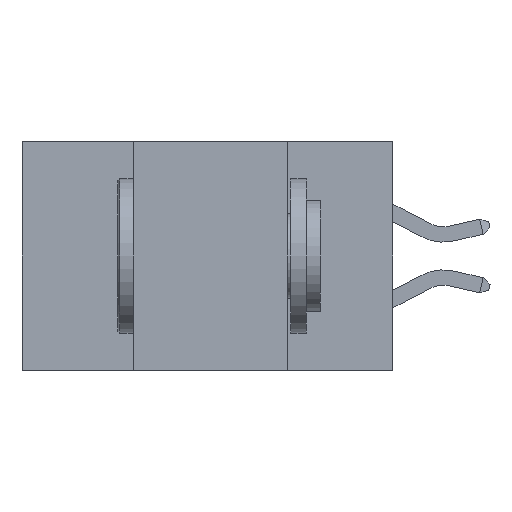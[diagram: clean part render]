
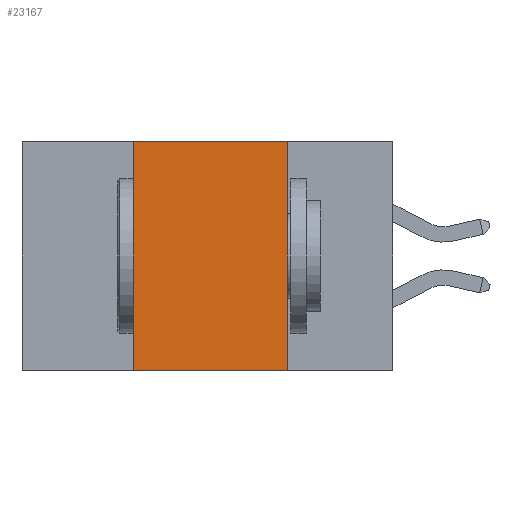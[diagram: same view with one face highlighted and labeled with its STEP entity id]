
A CAD part, left-side view. The second image highlights one B-rep face of the part: STEP entity #23167.
In plain terms, the highlighted planar face has unit normal (-1, 0, 0).
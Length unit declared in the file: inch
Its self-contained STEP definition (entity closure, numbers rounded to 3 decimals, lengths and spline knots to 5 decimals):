
#390 = EDGE_CURVE ( 'NONE', #35558, #11624, #39982, .T. ) ;
#1062 = VERTEX_POINT ( 'NONE', #30200 ) ;
#2316 = DIRECTION ( 'NONE',  ( 0., 0., -1. ) ) ;
#5757 = ORIENTED_EDGE ( 'NONE', *, *, #390, .F. ) ;
#5791 = PLANE ( 'NONE',  #6320 ) ;
#6320 = AXIS2_PLACEMENT_3D ( 'NONE', #9285, #32191, #12576 ) ;
#6738 = DIRECTION ( 'NONE',  ( 0., -1., 0. ) ) ;
#9285 = CARTESIAN_POINT ( 'NONE',  ( 0., 0.6, 0. ) ) ;
#10942 = EDGE_LOOP ( 'NONE', ( #28125, #5757, #19168, #29749 ) ) ;
#11624 = VERTEX_POINT ( 'NONE', #15081 ) ;
#11671 = CARTESIAN_POINT ( 'NONE',  ( 0., 0.17, -0.37 ) ) ;
#12576 = DIRECTION ( 'NONE',  ( 0., 0., -1. ) ) ;
#13021 = DIRECTION ( 'NONE',  ( 0., 0., 1. ) ) ;
#13224 = CARTESIAN_POINT ( 'NONE',  ( 0., 0.6, -0.37 ) ) ;
#13572 = CARTESIAN_POINT ( 'NONE',  ( 0., 0.6, 0. ) ) ;
#15081 = CARTESIAN_POINT ( 'NONE',  ( 0., 0.17, 0. ) ) ;
#15879 = VECTOR ( 'NONE', #13021, 39.37008 ) ;
#17072 = VECTOR ( 'NONE', #6738, 39.37008 ) ;
#17539 = VERTEX_POINT ( 'NONE', #11671 ) ;
#17560 = CARTESIAN_POINT ( 'NONE',  ( 0., 0.42, 0. ) ) ;
#19168 = ORIENTED_EDGE ( 'NONE', *, *, #20174, .F. ) ;
#19744 = CARTESIAN_POINT ( 'NONE',  ( 0., 0.42, 0. ) ) ;
#20174 = EDGE_CURVE ( 'NONE', #1062, #35558, #22017, .T. ) ;
#21080 = VECTOR ( 'NONE', #2316, 39.37008 ) ;
#22017 = LINE ( 'NONE', #19744, #15879 ) ;
#23167 = ADVANCED_FACE ( 'NONE', ( #33604 ), #5791, .F. ) ;
#28125 = ORIENTED_EDGE ( 'NONE', *, *, #39306, .F. ) ;
#29186 = VECTOR ( 'NONE', #33602, 39.37008 ) ;
#29749 = ORIENTED_EDGE ( 'NONE', *, *, #37909, .T. ) ;
#30200 = CARTESIAN_POINT ( 'NONE',  ( 0., 0.42, -0.37 ) ) ;
#32191 = DIRECTION ( 'NONE',  ( 1., 0., 0. ) ) ;
#33602 = DIRECTION ( 'NONE',  ( 0., -1., 0. ) ) ;
#33604 = FACE_OUTER_BOUND ( 'NONE', #10942, .T. ) ;
#35558 = VERTEX_POINT ( 'NONE', #17560 ) ;
#37909 = EDGE_CURVE ( 'NONE', #1062, #17539, #39093, .T. ) ;
#39093 = LINE ( 'NONE', #13224, #17072 ) ;
#39306 = EDGE_CURVE ( 'NONE', #11624, #17539, #41578, .T. ) ;
#39982 = LINE ( 'NONE', #13572, #29186 ) ;
#41578 = LINE ( 'NONE', #41869, #21080 ) ;
#41869 = CARTESIAN_POINT ( 'NONE',  ( 0., 0.17, 0. ) ) ;
